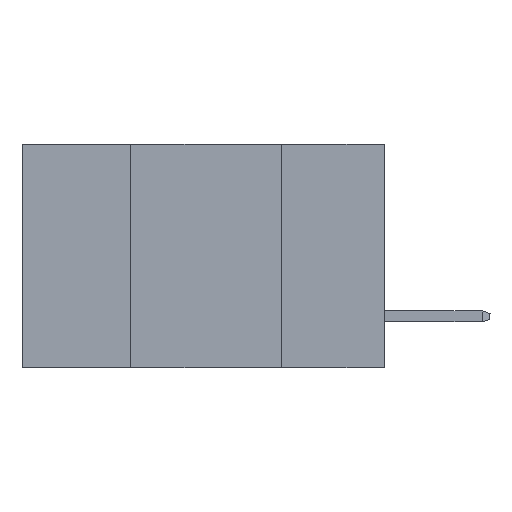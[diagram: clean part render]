
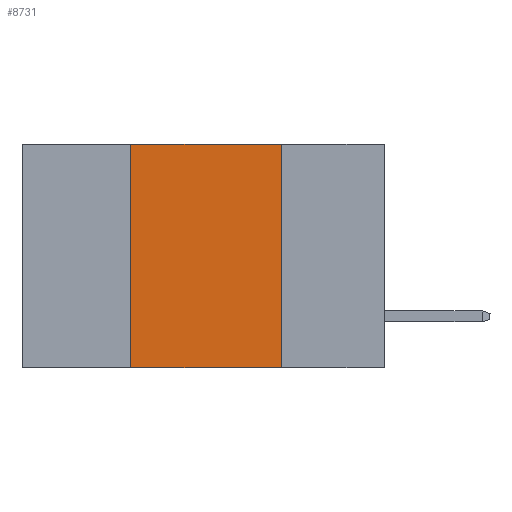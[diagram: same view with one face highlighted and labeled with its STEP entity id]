
A CAD part, left-side view. The second image highlights one B-rep face of the part: STEP entity #8731.
In plain terms, the highlighted planar face has unit normal (-1, 0, 0).
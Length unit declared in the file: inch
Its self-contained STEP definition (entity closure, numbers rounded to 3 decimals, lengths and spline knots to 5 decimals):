
#1063 = EDGE_CURVE ( 'NONE', #11742, #12806, #5493, .T. ) ;
#2717 = EDGE_LOOP ( 'NONE', ( #11394, #6719, #4499, #7015 ) ) ;
#2757 = DIRECTION ( 'NONE',  ( 0., 0., -1. ) ) ;
#2853 = CARTESIAN_POINT ( 'NONE',  ( 0., 0.17, -0.37 ) ) ;
#3320 = CARTESIAN_POINT ( 'NONE',  ( 0., 0.17, 0. ) ) ;
#3342 = DIRECTION ( 'NONE',  ( 0., -1., 0. ) ) ;
#3784 = VERTEX_POINT ( 'NONE', #3320 ) ;
#4499 = ORIENTED_EDGE ( 'NONE', *, *, #5112, .F. ) ;
#5112 = EDGE_CURVE ( 'NONE', #11742, #6490, #16251, .T. ) ;
#5493 = LINE ( 'NONE', #6906, #14885 ) ;
#6280 = DIRECTION ( 'NONE',  ( 1., 0., 0. ) ) ;
#6490 = VERTEX_POINT ( 'NONE', #9920 ) ;
#6719 = ORIENTED_EDGE ( 'NONE', *, *, #16036, .F. ) ;
#6906 = CARTESIAN_POINT ( 'NONE',  ( 0., 0.6, -0.37 ) ) ;
#7015 = ORIENTED_EDGE ( 'NONE', *, *, #1063, .T. ) ;
#8348 = EDGE_CURVE ( 'NONE', #3784, #12806, #14646, .T. ) ;
#8731 = ADVANCED_FACE ( 'NONE', ( #14208 ), #12777, .F. ) ;
#9560 = VECTOR ( 'NONE', #9999, 39.37008 ) ;
#9622 = VECTOR ( 'NONE', #15904, 39.37008 ) ;
#9920 = CARTESIAN_POINT ( 'NONE',  ( 0., 0.42, 0. ) ) ;
#9999 = DIRECTION ( 'NONE',  ( 0., 0., 1. ) ) ;
#11394 = ORIENTED_EDGE ( 'NONE', *, *, #8348, .F. ) ;
#11742 = VERTEX_POINT ( 'NONE', #14453 ) ;
#12777 = PLANE ( 'NONE',  #13865 ) ;
#12806 = VERTEX_POINT ( 'NONE', #15140 ) ;
#13585 = CARTESIAN_POINT ( 'NONE',  ( 0., 0.42, -0.37 ) ) ;
#13865 = AXIS2_PLACEMENT_3D ( 'NONE', #13958, #6280, #2757 ) ;
#13958 = CARTESIAN_POINT ( 'NONE',  ( 0., 0.6, 0. ) ) ;
#14208 = FACE_OUTER_BOUND ( 'NONE', #2717, .T. ) ;
#14453 = CARTESIAN_POINT ( 'NONE',  ( 0., 0.42, -0.37 ) ) ;
#14646 = LINE ( 'NONE', #2853, #9622 ) ;
#14715 = LINE ( 'NONE', #14800, #14779 ) ;
#14779 = VECTOR ( 'NONE', #3342, 39.37008 ) ;
#14800 = CARTESIAN_POINT ( 'NONE',  ( 0., 0.6, 0. ) ) ;
#14885 = VECTOR ( 'NONE', #15682, 39.37008 ) ;
#15140 = CARTESIAN_POINT ( 'NONE',  ( 0., 0.17, -0.37 ) ) ;
#15682 = DIRECTION ( 'NONE',  ( 0., -1., 0. ) ) ;
#15904 = DIRECTION ( 'NONE',  ( 0., 0., -1. ) ) ;
#16036 = EDGE_CURVE ( 'NONE', #6490, #3784, #14715, .T. ) ;
#16251 = LINE ( 'NONE', #13585, #9560 ) ;
